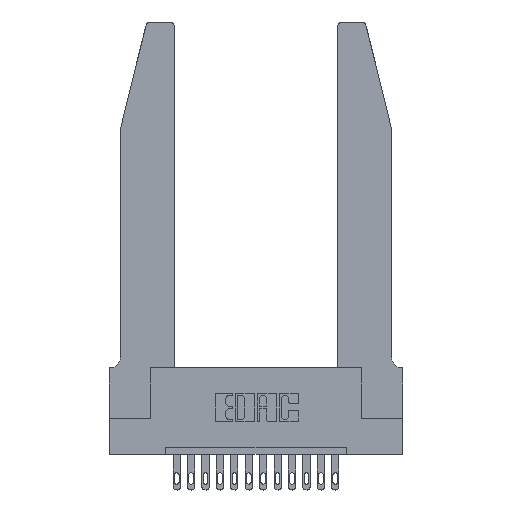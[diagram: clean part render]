
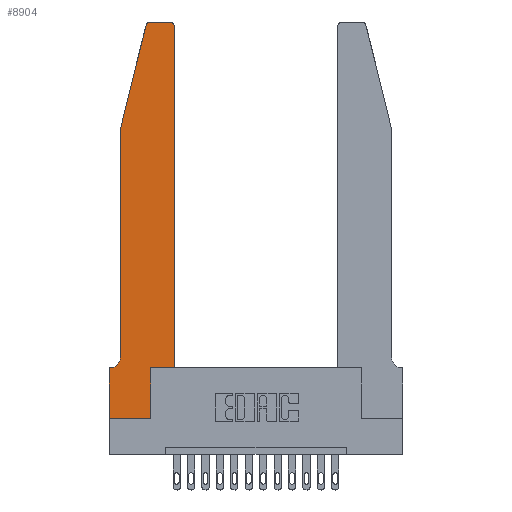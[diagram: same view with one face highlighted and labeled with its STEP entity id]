
A CAD part, top view. The second image highlights one B-rep face of the part: STEP entity #8904.
In plain terms, the highlighted planar face has unit normal (0, 0, 1).
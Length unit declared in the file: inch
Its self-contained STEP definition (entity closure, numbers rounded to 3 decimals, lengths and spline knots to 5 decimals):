
#25 = EDGE_CURVE ( 'NONE', #9019, #16368, #1266, .T. ) ;
#95 = DIRECTION ( 'NONE',  ( 1., 0., 0. ) ) ;
#109 = VERTEX_POINT ( 'NONE', #17086 ) ;
#445 = LINE ( 'NONE', #6692, #5410 ) ;
#469 = DIRECTION ( 'NONE',  ( -0.239, -0.971, 0. ) ) ;
#885 = EDGE_CURVE ( 'NONE', #8533, #9375, #9170, .T. ) ;
#954 = VECTOR ( 'NONE', #10444, 39.37008 ) ;
#988 = EDGE_CURVE ( 'NONE', #9747, #8533, #14301, .T. ) ;
#1246 = ORIENTED_EDGE ( 'NONE', *, *, #25, .T. ) ;
#1266 = LINE ( 'NONE', #2828, #11790 ) ;
#1445 = DIRECTION ( 'NONE',  ( 0., 1., 0. ) ) ;
#1479 = EDGE_LOOP ( 'NONE', ( #12841, #11076, #4061, #3664, #2840, #9322, #7933, #16939, #7372, #1246, #2911, #9299 ) ) ;
#1481 = AXIS2_PLACEMENT_3D ( 'NONE', #6111, #7497, #17049 ) ;
#1913 = AXIS2_PLACEMENT_3D ( 'NONE', #17590, #12061, #9466 ) ;
#2828 = CARTESIAN_POINT ( 'NONE',  ( 0.4505, 0.35, 0.37 ) ) ;
#2840 = ORIENTED_EDGE ( 'NONE', *, *, #988, .T. ) ;
#2911 = ORIENTED_EDGE ( 'NONE', *, *, #7509, .T. ) ;
#3246 = DIRECTION ( 'NONE',  ( 1., 0., 0. ) ) ;
#3306 = CIRCLE ( 'NONE', #1481, 0.03 ) ;
#3465 = CARTESIAN_POINT ( 'NONE',  ( 0.4505, 0.35, 0.37 ) ) ;
#3664 = ORIENTED_EDGE ( 'NONE', *, *, #15779, .T. ) ;
#4061 = ORIENTED_EDGE ( 'NONE', *, *, #7630, .T. ) ;
#4106 = LINE ( 'NONE', #15442, #14611 ) ;
#4128 = VERTEX_POINT ( 'NONE', #7661 ) ;
#4139 = VERTEX_POINT ( 'NONE', #6285 ) ;
#4160 = LINE ( 'NONE', #10784, #6972 ) ;
#4421 = CARTESIAN_POINT ( 'NONE',  ( 0.284, 2.75, 0.37 ) ) ;
#4985 = VECTOR ( 'NONE', #15842, 39.37008 ) ;
#5005 = CARTESIAN_POINT ( 'NONE',  ( 0.4505, 0.35, 0.37 ) ) ;
#5057 = CARTESIAN_POINT ( 'NONE',  ( 0.0755, 2., 0.37 ) ) ;
#5155 = EDGE_CURVE ( 'NONE', #109, #4128, #3306, .T. ) ;
#5264 = LINE ( 'NONE', #5057, #954 ) ;
#5410 = VECTOR ( 'NONE', #13417, 39.37008 ) ;
#5766 = DIRECTION ( 'NONE',  ( 0., 0., 1. ) ) ;
#5767 = CARTESIAN_POINT ( 'NONE',  ( 0., 0.35, 0.37 ) ) ;
#5823 = LINE ( 'NONE', #14316, #12097 ) ;
#6111 = CARTESIAN_POINT ( 'NONE',  ( 0.4205, 2.72, 0.37 ) ) ;
#6285 = CARTESIAN_POINT ( 'NONE',  ( 0.25487, 2.72718, 0.37 ) ) ;
#6641 = EDGE_CURVE ( 'NONE', #9375, #16044, #4160, .T. ) ;
#6692 = CARTESIAN_POINT ( 'NONE',  ( 0.2605, 2.75, 0.37 ) ) ;
#6972 = VECTOR ( 'NONE', #12185, 39.37008 ) ;
#7372 = ORIENTED_EDGE ( 'NONE', *, *, #12153, .T. ) ;
#7497 = DIRECTION ( 'NONE',  ( 0., 0., 1. ) ) ;
#7509 = EDGE_CURVE ( 'NONE', #16368, #109, #8648, .T. ) ;
#7630 = EDGE_CURVE ( 'NONE', #4139, #10340, #5823, .T. ) ;
#7656 = EDGE_CURVE ( 'NONE', #16044, #13004, #4106, .T. ) ;
#7661 = CARTESIAN_POINT ( 'NONE',  ( 0.4205, 2.75, 0.37 ) ) ;
#7827 = VECTOR ( 'NONE', #1445, 39.37008 ) ;
#7933 = ORIENTED_EDGE ( 'NONE', *, *, #6641, .T. ) ;
#8160 = CARTESIAN_POINT ( 'NONE',  ( 0.2865, 0., 0.37 ) ) ;
#8533 = VERTEX_POINT ( 'NONE', #13139 ) ;
#8578 = DIRECTION ( 'NONE',  ( 1., 0., 0. ) ) ;
#8648 = LINE ( 'NONE', #5005, #4985 ) ;
#8904 = ADVANCED_FACE ( 'NONE', ( #11160 ), #13995, .T. ) ;
#8986 = CARTESIAN_POINT ( 'NONE',  ( 0.0755, 0.42, 0.37 ) ) ;
#9019 = VERTEX_POINT ( 'NONE', #14754 ) ;
#9170 = LINE ( 'NONE', #10186, #16001 ) ;
#9299 = ORIENTED_EDGE ( 'NONE', *, *, #5155, .T. ) ;
#9322 = ORIENTED_EDGE ( 'NONE', *, *, #885, .T. ) ;
#9375 = VERTEX_POINT ( 'NONE', #17618 ) ;
#9466 = DIRECTION ( 'NONE',  ( -1., 0., 0. ) ) ;
#9747 = VERTEX_POINT ( 'NONE', #8986 ) ;
#10186 = CARTESIAN_POINT ( 'NONE',  ( 0.0755, 0.35, 0.37 ) ) ;
#10340 = VERTEX_POINT ( 'NONE', #12908 ) ;
#10444 = DIRECTION ( 'NONE',  ( 0., -1., 0. ) ) ;
#10784 = CARTESIAN_POINT ( 'NONE',  ( 0., 0., 0.37 ) ) ;
#10795 = CIRCLE ( 'NONE', #15267, 0.03 ) ;
#10857 = VERTEX_POINT ( 'NONE', #4421 ) ;
#11076 = ORIENTED_EDGE ( 'NONE', *, *, #17392, .T. ) ;
#11102 = CARTESIAN_POINT ( 'NONE',  ( 0., 0., 0.37 ) ) ;
#11120 = CARTESIAN_POINT ( 'NONE',  ( 0.2865, 0.35, 0.37 ) ) ;
#11160 = FACE_OUTER_BOUND ( 'NONE', #1479, .T. ) ;
#11790 = VECTOR ( 'NONE', #95, 39.37008 ) ;
#12061 = DIRECTION ( 'NONE',  ( 0., 0., -1. ) ) ;
#12097 = VECTOR ( 'NONE', #469, 39.37008 ) ;
#12153 = EDGE_CURVE ( 'NONE', #13004, #9019, #16819, .T. ) ;
#12185 = DIRECTION ( 'NONE',  ( 0., -1., 0. ) ) ;
#12841 = ORIENTED_EDGE ( 'NONE', *, *, #17774, .T. ) ;
#12908 = CARTESIAN_POINT ( 'NONE',  ( 0.0755, 2., 0.37 ) ) ;
#13004 = VERTEX_POINT ( 'NONE', #8160 ) ;
#13139 = CARTESIAN_POINT ( 'NONE',  ( 0.0055, 0.35, 0.37 ) ) ;
#13390 = DIRECTION ( 'NONE',  ( -1., 0., 0. ) ) ;
#13417 = DIRECTION ( 'NONE',  ( -1., 0., 0. ) ) ;
#13889 = DIRECTION ( 'NONE',  ( 1., 0., 0. ) ) ;
#13995 = PLANE ( 'NONE',  #16692 ) ;
#14301 = CIRCLE ( 'NONE', #1913, 0.07 ) ;
#14316 = CARTESIAN_POINT ( 'NONE',  ( 0.0755, 2., 0.37 ) ) ;
#14611 = VECTOR ( 'NONE', #8578, 39.37008 ) ;
#14754 = CARTESIAN_POINT ( 'NONE',  ( 0.2865, 0.35, 0.37 ) ) ;
#15267 = AXIS2_PLACEMENT_3D ( 'NONE', #15297, #5766, #13889 ) ;
#15297 = CARTESIAN_POINT ( 'NONE',  ( 0.284, 2.72, 0.37 ) ) ;
#15442 = CARTESIAN_POINT ( 'NONE',  ( 0., 0., 0.37 ) ) ;
#15779 = EDGE_CURVE ( 'NONE', #10340, #9747, #5264, .T. ) ;
#15825 = DIRECTION ( 'NONE',  ( 0., 0., 1. ) ) ;
#15842 = DIRECTION ( 'NONE',  ( 0., 1., 0. ) ) ;
#16001 = VECTOR ( 'NONE', #13390, 39.37008 ) ;
#16044 = VERTEX_POINT ( 'NONE', #11102 ) ;
#16368 = VERTEX_POINT ( 'NONE', #3465 ) ;
#16692 = AXIS2_PLACEMENT_3D ( 'NONE', #5767, #15825, #3246 ) ;
#16819 = LINE ( 'NONE', #11120, #7827 ) ;
#16939 = ORIENTED_EDGE ( 'NONE', *, *, #7656, .T. ) ;
#17049 = DIRECTION ( 'NONE',  ( 1., 0., 0. ) ) ;
#17086 = CARTESIAN_POINT ( 'NONE',  ( 0.4505, 2.72, 0.37 ) ) ;
#17392 = EDGE_CURVE ( 'NONE', #10857, #4139, #10795, .T. ) ;
#17590 = CARTESIAN_POINT ( 'NONE',  ( 0.0055, 0.42, 0.37 ) ) ;
#17618 = CARTESIAN_POINT ( 'NONE',  ( 0., 0.35, 0.37 ) ) ;
#17774 = EDGE_CURVE ( 'NONE', #4128, #10857, #445, .T. ) ;
